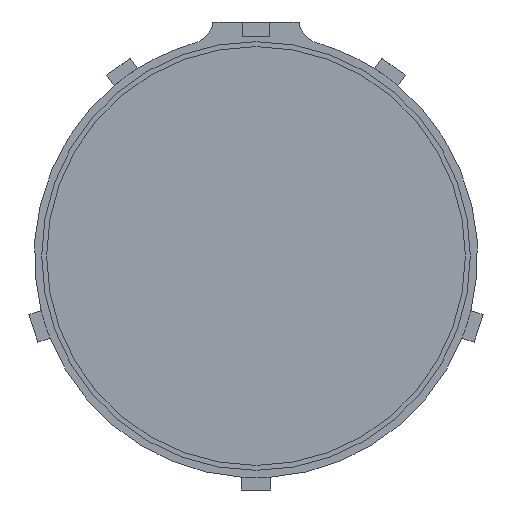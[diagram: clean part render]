
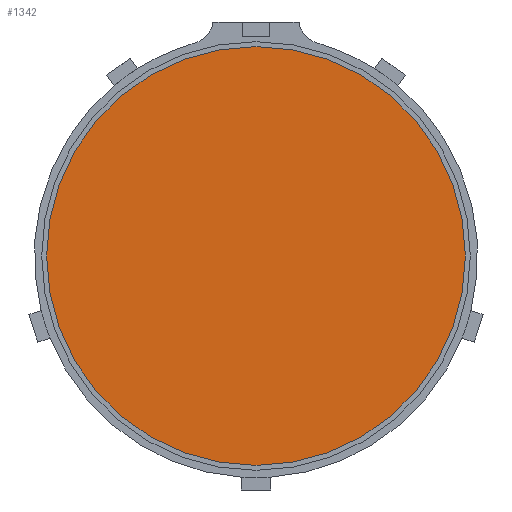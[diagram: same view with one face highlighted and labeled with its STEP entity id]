
A CAD part, front view. The second image highlights one B-rep face of the part: STEP entity #1342.
In plain terms, the highlighted planar face has unit normal (0, -1, 0).
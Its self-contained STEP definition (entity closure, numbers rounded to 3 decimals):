
#5 = EDGE_CURVE ( 'NONE', #2355, #1963, #1970, .T. ) ;
#99 = FACE_OUTER_BOUND ( 'NONE', #1070, .T. ) ;
#384 = ORIENTED_EDGE ( 'NONE', *, *, #5, .F. ) ;
#649 = CARTESIAN_POINT ( 'NONE',  ( 0., 70., 0. ) ) ;
#702 = DIRECTION ( 'NONE',  ( 0., 0., 1. ) ) ;
#856 = CARTESIAN_POINT ( 'NONE',  ( 0., 70., 0. ) ) ;
#863 = CARTESIAN_POINT ( 'NONE',  ( 0., 70., 85. ) ) ;
#901 = CARTESIAN_POINT ( 'NONE',  ( 0., 70., -85. ) ) ;
#924 = AXIS2_PLACEMENT_3D ( 'NONE', #649, #1230, #1456 ) ;
#1070 = EDGE_LOOP ( 'NONE', ( #1208, #384 ) ) ;
#1208 = ORIENTED_EDGE ( 'NONE', *, *, #1478, .F. ) ;
#1230 = DIRECTION ( 'NONE',  ( 0., 1., 0. ) ) ;
#1287 = CIRCLE ( 'NONE', #924, 85. ) ;
#1342 = ADVANCED_FACE ( 'NONE', ( #99 ), #2217, .F. ) ;
#1448 = DIRECTION ( 'NONE',  ( 0., 1., 0. ) ) ;
#1456 = DIRECTION ( 'NONE',  ( 0., 0., 1. ) ) ;
#1478 = EDGE_CURVE ( 'NONE', #1963, #2355, #1287, .T. ) ;
#1585 = DIRECTION ( 'NONE',  ( 0., 1., 0. ) ) ;
#1963 = VERTEX_POINT ( 'NONE', #901 ) ;
#1970 = CIRCLE ( 'NONE', #2382, 85. ) ;
#2112 = DIRECTION ( 'NONE',  ( 0., 0., 1. ) ) ;
#2217 = PLANE ( 'NONE',  #2332 ) ;
#2224 = CARTESIAN_POINT ( 'NONE',  ( 0., 70., 0. ) ) ;
#2332 = AXIS2_PLACEMENT_3D ( 'NONE', #2224, #1448, #702 ) ;
#2355 = VERTEX_POINT ( 'NONE', #863 ) ;
#2382 = AXIS2_PLACEMENT_3D ( 'NONE', #856, #1585, #2112 ) ;
